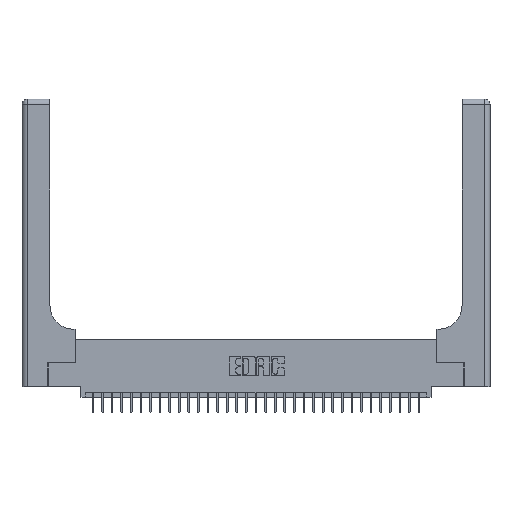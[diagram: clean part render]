
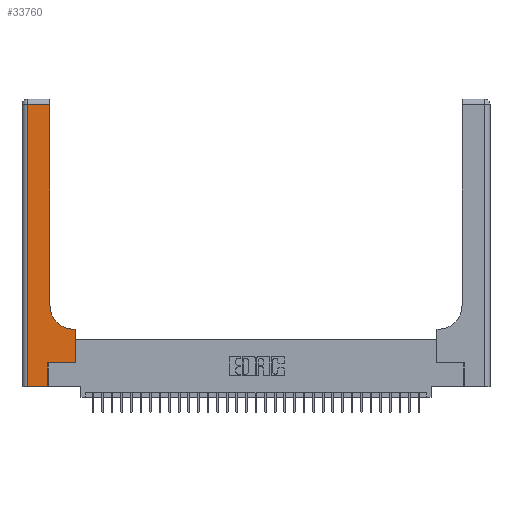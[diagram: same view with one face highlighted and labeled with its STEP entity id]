
A CAD part, top view. The second image highlights one B-rep face of the part: STEP entity #33760.
In plain terms, the highlighted planar face has unit normal (0, 0, 1).
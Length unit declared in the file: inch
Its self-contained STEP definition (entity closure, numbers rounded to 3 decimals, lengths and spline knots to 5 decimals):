
#1702 = EDGE_CURVE ( 'NONE', #30231, #31967, #26164, .T. ) ;
#2026 = CARTESIAN_POINT ( 'NONE',  ( 0.5585, 0.25, 0.37 ) ) ;
#2598 = LINE ( 'NONE', #23442, #27495 ) ;
#2602 = ORIENTED_EDGE ( 'NONE', *, *, #30477, .T. ) ;
#2637 = AXIS2_PLACEMENT_3D ( 'NONE', #7699, #33639, #31438 ) ;
#3487 = CARTESIAN_POINT ( 'NONE',  ( 0.5415, 0.6, 0.37 ) ) ;
#3819 = LINE ( 'NONE', #22966, #15285 ) ;
#3859 = VECTOR ( 'NONE', #17898, 39.37008 ) ;
#4683 = CARTESIAN_POINT ( 'NONE',  ( 0.06, 3., 0.37 ) ) ;
#5234 = VECTOR ( 'NONE', #18914, 39.37008 ) ;
#5414 = DIRECTION ( 'NONE',  ( 1., 0., 0. ) ) ;
#5911 = ORIENTED_EDGE ( 'NONE', *, *, #7666, .T. ) ;
#7217 = ORIENTED_EDGE ( 'NONE', *, *, #25139, .T. ) ;
#7378 = DIRECTION ( 'NONE',  ( 0., 1., 0. ) ) ;
#7539 = LINE ( 'NONE', #4683, #3859 ) ;
#7666 = EDGE_CURVE ( 'NONE', #23026, #9865, #8083, .T. ) ;
#7699 = CARTESIAN_POINT ( 'NONE',  ( 0.5415, 0.85, 0.37 ) ) ;
#7888 = DIRECTION ( 'NONE',  ( 0., 0., -1. ) ) ;
#8083 = LINE ( 'NONE', #21533, #5234 ) ;
#9407 = VECTOR ( 'NONE', #7378, 39.37008 ) ;
#9501 = VERTEX_POINT ( 'NONE', #11631 ) ;
#9865 = VERTEX_POINT ( 'NONE', #15864 ) ;
#10040 = EDGE_CURVE ( 'NONE', #9865, #30301, #26186, .T. ) ;
#10358 = ORIENTED_EDGE ( 'NONE', *, *, #1702, .T. ) ;
#10387 = CARTESIAN_POINT ( 'NONE',  ( 0., 3., 0.37 ) ) ;
#10659 = LINE ( 'NONE', #2026, #9407 ) ;
#11250 = CIRCLE ( 'NONE', #2637, 0.25 ) ;
#11631 = CARTESIAN_POINT ( 'NONE',  ( 0.269, 0.25, 0.37 ) ) ;
#11702 = CARTESIAN_POINT ( 'NONE',  ( 0.5585, 0.25, 0.37 ) ) ;
#11825 = EDGE_CURVE ( 'NONE', #33332, #9501, #3819, .T. ) ;
#12252 = CARTESIAN_POINT ( 'NONE',  ( 0.5585, 0.6, 0.37 ) ) ;
#12604 = CARTESIAN_POINT ( 'NONE',  ( 0., 2.94, 0.37 ) ) ;
#14309 = VECTOR ( 'NONE', #18189, 39.37008 ) ;
#15285 = VECTOR ( 'NONE', #25242, 39.37008 ) ;
#15428 = PLANE ( 'NONE',  #33073 ) ;
#15864 = CARTESIAN_POINT ( 'NONE',  ( 0.2915, 2.94, 0.37 ) ) ;
#16451 = ORIENTED_EDGE ( 'NONE', *, *, #32338, .T. ) ;
#17526 = EDGE_CURVE ( 'NONE', #30301, #24022, #7539, .T. ) ;
#17898 = DIRECTION ( 'NONE',  ( 0., -1., 0. ) ) ;
#18189 = DIRECTION ( 'NONE',  ( -1., 0., 0. ) ) ;
#18373 = ORIENTED_EDGE ( 'NONE', *, *, #25489, .T. ) ;
#18914 = DIRECTION ( 'NONE',  ( 0., 1., 0. ) ) ;
#19455 = CARTESIAN_POINT ( 'NONE',  ( 0., 0., 0.37 ) ) ;
#19644 = VERTEX_POINT ( 'NONE', #11702 ) ;
#21440 = ORIENTED_EDGE ( 'NONE', *, *, #10040, .T. ) ;
#21533 = CARTESIAN_POINT ( 'NONE',  ( 0.2915, 3., 0.37 ) ) ;
#22679 = FACE_OUTER_BOUND ( 'NONE', #24040, .T. ) ;
#22966 = CARTESIAN_POINT ( 'NONE',  ( 0.269, 0., 0.37 ) ) ;
#23026 = VERTEX_POINT ( 'NONE', #27665 ) ;
#23108 = CARTESIAN_POINT ( 'NONE',  ( 0.06, 2.94, 0.37 ) ) ;
#23164 = DIRECTION ( 'NONE',  ( -1., 0., 0. ) ) ;
#23442 = CARTESIAN_POINT ( 'NONE',  ( 0.269, 0.25, 0.37 ) ) ;
#24022 = VERTEX_POINT ( 'NONE', #28139 ) ;
#24040 = EDGE_LOOP ( 'NONE', ( #5911, #21440, #32237, #18373, #32158, #2602, #7217, #10358, #16451 ) ) ;
#25139 = EDGE_CURVE ( 'NONE', #19644, #30231, #10659, .T. ) ;
#25242 = DIRECTION ( 'NONE',  ( 0., 1., 0. ) ) ;
#25489 = EDGE_CURVE ( 'NONE', #24022, #33332, #27806, .T. ) ;
#25606 = DIRECTION ( 'NONE',  ( -1., 0., 0. ) ) ;
#26164 = LINE ( 'NONE', #33719, #31051 ) ;
#26186 = LINE ( 'NONE', #12604, #14309 ) ;
#27495 = VECTOR ( 'NONE', #5414, 39.37008 ) ;
#27665 = CARTESIAN_POINT ( 'NONE',  ( 0.2915, 0.85, 0.37 ) ) ;
#27806 = LINE ( 'NONE', #19455, #29023 ) ;
#28139 = CARTESIAN_POINT ( 'NONE',  ( 0.06, 0., 0.37 ) ) ;
#29023 = VECTOR ( 'NONE', #32362, 39.37008 ) ;
#30231 = VERTEX_POINT ( 'NONE', #12252 ) ;
#30301 = VERTEX_POINT ( 'NONE', #23108 ) ;
#30477 = EDGE_CURVE ( 'NONE', #9501, #19644, #2598, .T. ) ;
#31051 = VECTOR ( 'NONE', #25606, 39.37008 ) ;
#31438 = DIRECTION ( 'NONE',  ( 1., 0., 0. ) ) ;
#31967 = VERTEX_POINT ( 'NONE', #3487 ) ;
#32158 = ORIENTED_EDGE ( 'NONE', *, *, #11825, .T. ) ;
#32209 = CARTESIAN_POINT ( 'NONE',  ( 0.269, 0., 0.37 ) ) ;
#32237 = ORIENTED_EDGE ( 'NONE', *, *, #17526, .T. ) ;
#32338 = EDGE_CURVE ( 'NONE', #31967, #23026, #11250, .T. ) ;
#32362 = DIRECTION ( 'NONE',  ( 1., 0., 0. ) ) ;
#33073 = AXIS2_PLACEMENT_3D ( 'NONE', #10387, #7888, #23164 ) ;
#33332 = VERTEX_POINT ( 'NONE', #32209 ) ;
#33639 = DIRECTION ( 'NONE',  ( 0., 0., -1. ) ) ;
#33719 = CARTESIAN_POINT ( 'NONE',  ( 0.2915, 0.6, 0.37 ) ) ;
#33760 = ADVANCED_FACE ( 'NONE', ( #22679 ), #15428, .F. ) ;
